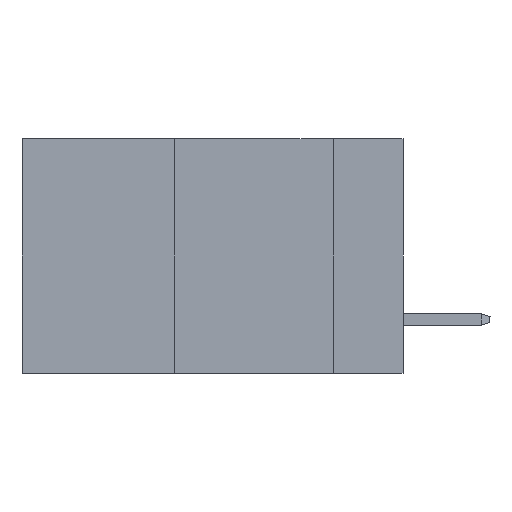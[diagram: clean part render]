
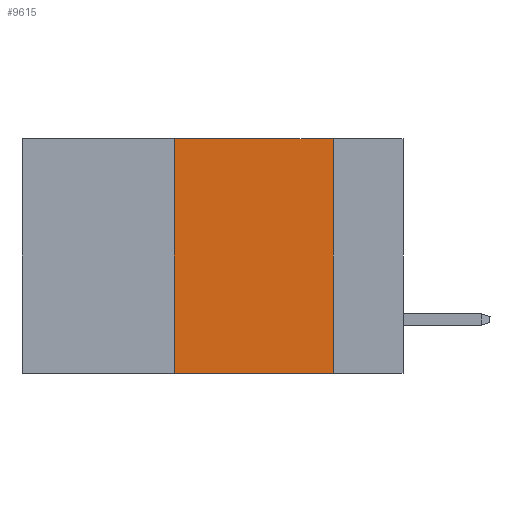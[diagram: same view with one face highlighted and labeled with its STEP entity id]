
A CAD part, left-side view. The second image highlights one B-rep face of the part: STEP entity #9615.
In plain terms, the highlighted planar face has unit normal (-1, 0, 0).
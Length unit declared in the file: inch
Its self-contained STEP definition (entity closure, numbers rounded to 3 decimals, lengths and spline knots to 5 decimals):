
#1434 = VERTEX_POINT ( 'NONE', #31793 ) ;
#2044 = EDGE_CURVE ( 'NONE', #22080, #11767, #3538, .T. ) ;
#2230 = AXIS2_PLACEMENT_3D ( 'NONE', #14817, #23372, #32022 ) ;
#3538 = LINE ( 'NONE', #34283, #5418 ) ;
#3882 = ORIENTED_EDGE ( 'NONE', *, *, #15750, .T. ) ;
#4811 = VECTOR ( 'NONE', #34567, 39.37008 ) ;
#5418 = VECTOR ( 'NONE', #15111, 39.37008 ) ;
#6552 = CARTESIAN_POINT ( 'NONE',  ( 0., 0.11, 0. ) ) ;
#7506 = LINE ( 'NONE', #18007, #25714 ) ;
#7948 = EDGE_CURVE ( 'NONE', #11767, #1434, #16808, .T. ) ;
#8180 = ORIENTED_EDGE ( 'NONE', *, *, #2044, .F. ) ;
#8319 = DIRECTION ( 'NONE',  ( 0., -1., 0. ) ) ;
#9615 = ADVANCED_FACE ( 'NONE', ( #29220 ), #34721, .F. ) ;
#9762 = VERTEX_POINT ( 'NONE', #18818 ) ;
#10333 = CARTESIAN_POINT ( 'NONE',  ( 0., 0.36, -0.37 ) ) ;
#10692 = VECTOR ( 'NONE', #8319, 39.37008 ) ;
#11767 = VERTEX_POINT ( 'NONE', #21494 ) ;
#14069 = ORIENTED_EDGE ( 'NONE', *, *, #7948, .F. ) ;
#14817 = CARTESIAN_POINT ( 'NONE',  ( 0., 0.6, 0. ) ) ;
#15111 = DIRECTION ( 'NONE',  ( 0., 0., 1. ) ) ;
#15750 = EDGE_CURVE ( 'NONE', #22080, #9762, #7506, .T. ) ;
#16808 = LINE ( 'NONE', #16983, #10692 ) ;
#16983 = CARTESIAN_POINT ( 'NONE',  ( 0., 0.6, 0. ) ) ;
#17821 = ORIENTED_EDGE ( 'NONE', *, *, #31248, .F. ) ;
#18007 = CARTESIAN_POINT ( 'NONE',  ( 0., 0.6, -0.37 ) ) ;
#18818 = CARTESIAN_POINT ( 'NONE',  ( 0., 0.11, -0.37 ) ) ;
#20512 = LINE ( 'NONE', #6552, #4811 ) ;
#21494 = CARTESIAN_POINT ( 'NONE',  ( 0., 0.36, 0. ) ) ;
#22080 = VERTEX_POINT ( 'NONE', #10333 ) ;
#23372 = DIRECTION ( 'NONE',  ( 1., 0., 0. ) ) ;
#25714 = VECTOR ( 'NONE', #26743, 39.37008 ) ;
#26743 = DIRECTION ( 'NONE',  ( 0., -1., 0. ) ) ;
#27343 = EDGE_LOOP ( 'NONE', ( #17821, #14069, #8180, #3882 ) ) ;
#29220 = FACE_OUTER_BOUND ( 'NONE', #27343, .T. ) ;
#31248 = EDGE_CURVE ( 'NONE', #1434, #9762, #20512, .T. ) ;
#31793 = CARTESIAN_POINT ( 'NONE',  ( 0., 0.11, 0. ) ) ;
#32022 = DIRECTION ( 'NONE',  ( 0., 0., -1. ) ) ;
#34283 = CARTESIAN_POINT ( 'NONE',  ( 0., 0.36, 0. ) ) ;
#34567 = DIRECTION ( 'NONE',  ( 0., 0., -1. ) ) ;
#34721 = PLANE ( 'NONE',  #2230 ) ;
